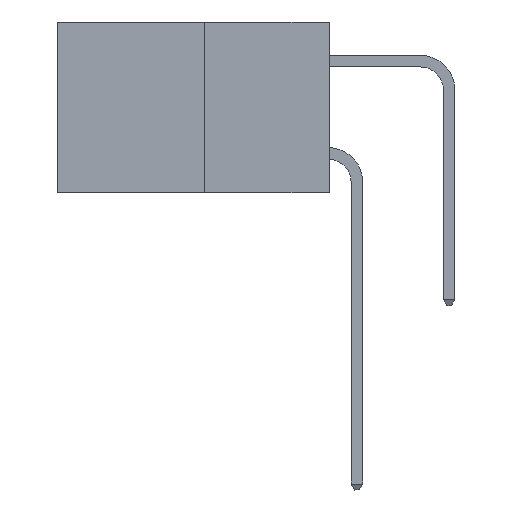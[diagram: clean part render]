
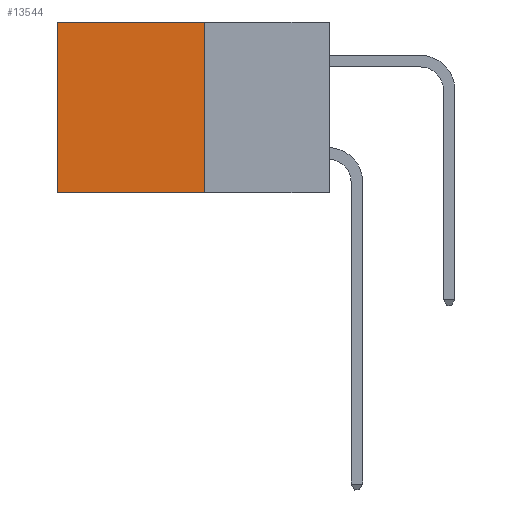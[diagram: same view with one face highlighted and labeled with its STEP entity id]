
A CAD part, left-side view. The second image highlights one B-rep face of the part: STEP entity #13544.
In plain terms, the highlighted planar face has unit normal (-1, 0, 0).
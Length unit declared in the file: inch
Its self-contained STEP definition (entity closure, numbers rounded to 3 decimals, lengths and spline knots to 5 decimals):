
#588 = LINE ( 'NONE', #8819, #10184 ) ;
#700 = VECTOR ( 'NONE', #13140, 39.37008 ) ;
#732 = DIRECTION ( 'NONE',  ( 0., 1., 0. ) ) ;
#841 = CARTESIAN_POINT ( 'NONE',  ( 0.277, 0.59, 0. ) ) ;
#1707 = EDGE_CURVE ( 'NONE', #1947, #13828, #14269, .T. ) ;
#1818 = DIRECTION ( 'NONE',  ( 1., 0., 0. ) ) ;
#1947 = VERTEX_POINT ( 'NONE', #841 ) ;
#2045 = DIRECTION ( 'NONE',  ( 0., 1., 0. ) ) ;
#2346 = CARTESIAN_POINT ( 'NONE',  ( 0.277, 0.59, -0.37 ) ) ;
#2967 = CARTESIAN_POINT ( 'NONE',  ( 0.277, 0.27, 0. ) ) ;
#4305 = VERTEX_POINT ( 'NONE', #2967 ) ;
#5179 = FACE_OUTER_BOUND ( 'NONE', #7999, .T. ) ;
#5720 = CARTESIAN_POINT ( 'NONE',  ( 0.277, 0.27, -0.37 ) ) ;
#7851 = VECTOR ( 'NONE', #732, 39.37008 ) ;
#7999 = EDGE_LOOP ( 'NONE', ( #13654, #8361, #11568, #14814 ) ) ;
#8361 = ORIENTED_EDGE ( 'NONE', *, *, #11783, .F. ) ;
#8819 = CARTESIAN_POINT ( 'NONE',  ( 0.277, 0.27, -0.37 ) ) ;
#9052 = VERTEX_POINT ( 'NONE', #11428 ) ;
#9332 = CARTESIAN_POINT ( 'NONE',  ( 0.277, 0.27, -0.37 ) ) ;
#9666 = EDGE_CURVE ( 'NONE', #4305, #9052, #588, .T. ) ;
#10098 = LINE ( 'NONE', #10762, #12959 ) ;
#10184 = VECTOR ( 'NONE', #14925, 39.37008 ) ;
#10536 = DIRECTION ( 'NONE',  ( 0., 0., -1. ) ) ;
#10762 = CARTESIAN_POINT ( 'NONE',  ( 0.277, 0.27, 0. ) ) ;
#11077 = LINE ( 'NONE', #5720, #7851 ) ;
#11428 = CARTESIAN_POINT ( 'NONE',  ( 0.277, 0.27, -0.37 ) ) ;
#11568 = ORIENTED_EDGE ( 'NONE', *, *, #9666, .F. ) ;
#11783 = EDGE_CURVE ( 'NONE', #9052, #13828, #11077, .T. ) ;
#12761 = CARTESIAN_POINT ( 'NONE',  ( 0.277, 0.59, -0.37 ) ) ;
#12943 = PLANE ( 'NONE',  #14121 ) ;
#12959 = VECTOR ( 'NONE', #2045, 39.37008 ) ;
#13026 = EDGE_CURVE ( 'NONE', #4305, #1947, #10098, .T. ) ;
#13140 = DIRECTION ( 'NONE',  ( 0., 0., -1. ) ) ;
#13544 = ADVANCED_FACE ( 'NONE', ( #5179 ), #12943, .F. ) ;
#13654 = ORIENTED_EDGE ( 'NONE', *, *, #1707, .T. ) ;
#13828 = VERTEX_POINT ( 'NONE', #2346 ) ;
#14121 = AXIS2_PLACEMENT_3D ( 'NONE', #9332, #1818, #10536 ) ;
#14269 = LINE ( 'NONE', #12761, #700 ) ;
#14814 = ORIENTED_EDGE ( 'NONE', *, *, #13026, .T. ) ;
#14925 = DIRECTION ( 'NONE',  ( 0., 0., -1. ) ) ;
